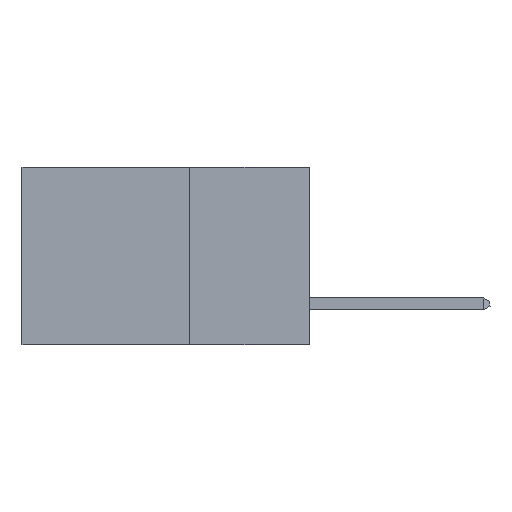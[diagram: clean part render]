
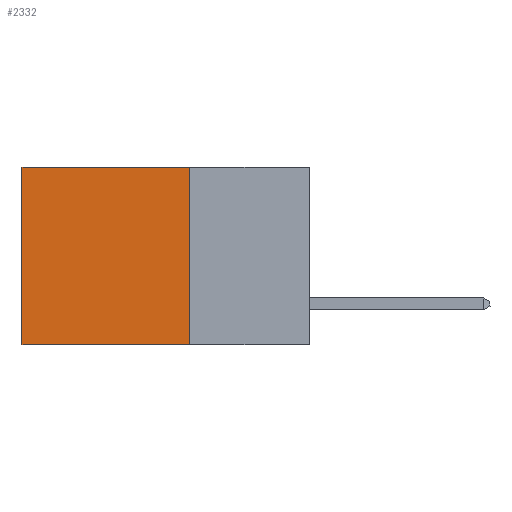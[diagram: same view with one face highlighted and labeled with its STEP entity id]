
A CAD part, left-side view. The second image highlights one B-rep face of the part: STEP entity #2332.
In plain terms, the highlighted planar face has unit normal (-1, 0, 0).
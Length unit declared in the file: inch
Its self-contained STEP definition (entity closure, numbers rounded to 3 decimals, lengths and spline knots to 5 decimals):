
#23 = EDGE_CURVE ( 'NONE', #7043, #7446, #11192, .T. ) ;
#129 = LINE ( 'NONE', #7776, #6780 ) ;
#393 = CARTESIAN_POINT ( 'NONE',  ( 0.2875, 0.25, 0. ) ) ;
#429 = CARTESIAN_POINT ( 'NONE',  ( 0.2875, 0.25, 0. ) ) ;
#1643 = VECTOR ( 'NONE', #7898, 39.37008 ) ;
#2332 = ADVANCED_FACE ( 'NONE', ( #10925 ), #9084, .F. ) ;
#3019 = CARTESIAN_POINT ( 'NONE',  ( 0.2875, 0.25, 0. ) ) ;
#3643 = VERTEX_POINT ( 'NONE', #6793 ) ;
#3680 = EDGE_LOOP ( 'NONE', ( #5986, #10346, #3966, #8402 ) ) ;
#3966 = ORIENTED_EDGE ( 'NONE', *, *, #9724, .F. ) ;
#4326 = LINE ( 'NONE', #5383, #1643 ) ;
#4392 = CARTESIAN_POINT ( 'NONE',  ( 0.2875, 0.25, -0.37 ) ) ;
#4634 = VECTOR ( 'NONE', #9189, 39.37008 ) ;
#4862 = CARTESIAN_POINT ( 'NONE',  ( 0.2875, 0.25, -0.37 ) ) ;
#5102 = DIRECTION ( 'NONE',  ( 1., 0., 0. ) ) ;
#5383 = CARTESIAN_POINT ( 'NONE',  ( 0.2875, 0.25, 0. ) ) ;
#5594 = EDGE_CURVE ( 'NONE', #5943, #3643, #9751, .T. ) ;
#5943 = VERTEX_POINT ( 'NONE', #4862 ) ;
#5986 = ORIENTED_EDGE ( 'NONE', *, *, #7745, .T. ) ;
#6154 = DIRECTION ( 'NONE',  ( 0., 0., -1. ) ) ;
#6586 = CARTESIAN_POINT ( 'NONE',  ( 0.2875, 0.6, 0. ) ) ;
#6780 = VECTOR ( 'NONE', #6154, 39.37008 ) ;
#6793 = CARTESIAN_POINT ( 'NONE',  ( 0.2875, 0.6, -0.37 ) ) ;
#7043 = VERTEX_POINT ( 'NONE', #393 ) ;
#7446 = VERTEX_POINT ( 'NONE', #6586 ) ;
#7745 = EDGE_CURVE ( 'NONE', #7446, #3643, #129, .T. ) ;
#7776 = CARTESIAN_POINT ( 'NONE',  ( 0.2875, 0.6, 0. ) ) ;
#7793 = AXIS2_PLACEMENT_3D ( 'NONE', #3019, #5102, #8992 ) ;
#7898 = DIRECTION ( 'NONE',  ( 0., 0., -1. ) ) ;
#8402 = ORIENTED_EDGE ( 'NONE', *, *, #23, .T. ) ;
#8992 = DIRECTION ( 'NONE',  ( 0., 0., -1. ) ) ;
#9084 = PLANE ( 'NONE',  #7793 ) ;
#9189 = DIRECTION ( 'NONE',  ( 0., 1., 0. ) ) ;
#9724 = EDGE_CURVE ( 'NONE', #7043, #5943, #4326, .T. ) ;
#9751 = LINE ( 'NONE', #4392, #11132 ) ;
#10346 = ORIENTED_EDGE ( 'NONE', *, *, #5594, .F. ) ;
#10925 = FACE_OUTER_BOUND ( 'NONE', #3680, .T. ) ;
#11000 = DIRECTION ( 'NONE',  ( 0., 1., 0. ) ) ;
#11132 = VECTOR ( 'NONE', #11000, 39.37008 ) ;
#11192 = LINE ( 'NONE', #429, #4634 ) ;
